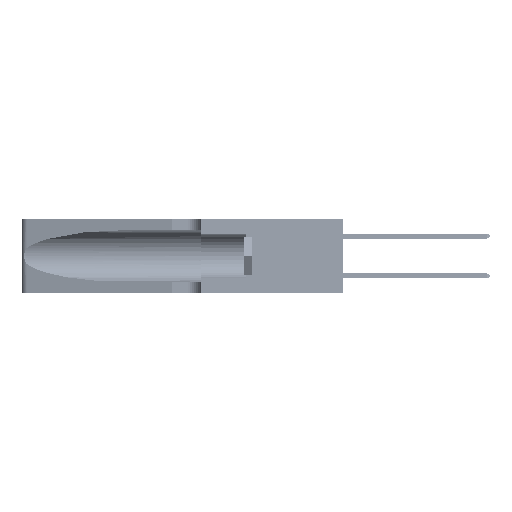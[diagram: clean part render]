
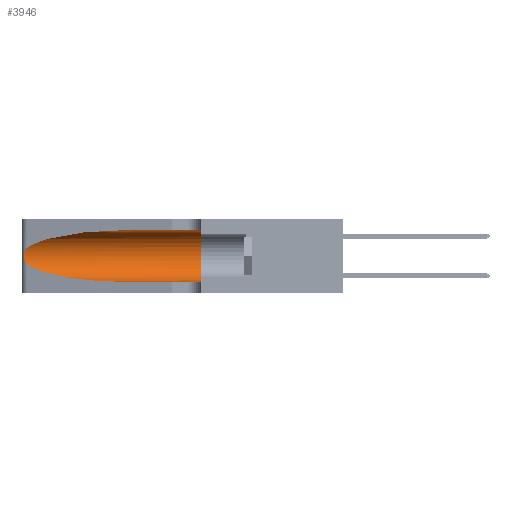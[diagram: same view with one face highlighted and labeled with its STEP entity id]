
A CAD part, left-side view. The second image highlights one B-rep face of the part: STEP entity #3946.
In plain terms, the highlighted cylindrical face has radius 3.308 mm (diameter 6.617 mm), a partial arc.
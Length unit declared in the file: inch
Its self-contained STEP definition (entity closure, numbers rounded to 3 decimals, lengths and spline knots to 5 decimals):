
#882 = DIRECTION ( 'NONE',  ( 0., -1., 0. ) ) ;
#1875 =( BOUNDED_CURVE ( )  B_SPLINE_CURVE ( 3, ( #15972, #15630, #47007, #19424 ),
 .UNSPECIFIED., .F., .F. ) 
 B_SPLINE_CURVE_WITH_KNOTS ( ( 4, 4 ),
 ( 3.44316, 4.71239 ),
 .UNSPECIFIED. ) 
 CURVE ( )  GEOMETRIC_REPRESENTATION_ITEM ( )  RATIONAL_B_SPLINE_CURVE ( ( 1., 0.87, 0.87, 1. ) ) 
 REPRESENTATION_ITEM ( '' )  );
#2103 = CARTESIAN_POINT ( 'NONE',  ( 0.1305, 1.61858, 0.05475 ) ) ;
#2652 = DIRECTION ( 'NONE',  ( 0., -1., 0. ) ) ;
#3429 = CARTESIAN_POINT ( 'NONE',  ( 0.1305, 0.72297, 0.31525 ) ) ;
#3946 = ADVANCED_FACE ( 'NONE', ( #29796 ), #18127, .F. ) ;
#4028 = EDGE_CURVE ( 'NONE', #24841, #21678, #39055, .T. ) ;
#4341 = CARTESIAN_POINT ( 'NONE',  ( 0.25487, 1.22718, 0.22369 ) ) ;
#4496 = VERTEX_POINT ( 'NONE', #13826 ) ;
#5015 = CARTESIAN_POINT ( 'NONE',  ( 0.25789, 1.23486, 0.15765 ) ) ;
#5177 = CARTESIAN_POINT ( 'NONE',  ( 0.1305, 1.61858, 0.31525 ) ) ;
#7983 = EDGE_CURVE ( 'NONE', #21678, #39551, #42183, .T. ) ;
#8445 = CARTESIAN_POINT ( 'NONE',  ( 0.26075, 1.23896, 0.178 ) ) ;
#8957 = CARTESIAN_POINT ( 'NONE',  ( 0.25854, 1.2359, 0.20912 ) ) ;
#11579 = CARTESIAN_POINT ( 'NONE',  ( 0.25487, 1.22718, 0.14631 ) ) ;
#12731 = EDGE_CURVE ( 'NONE', #25545, #4496, #20174, .T. ) ;
#12891 = CARTESIAN_POINT ( 'NONE',  ( 0.25487, 1.22718, 0.22369 ) ) ;
#12968 = CARTESIAN_POINT ( 'NONE',  ( 0.25487, 1.22718, 0.14631 ) ) ;
#13826 = CARTESIAN_POINT ( 'NONE',  ( 0.1305, 0.35, 0.05475 ) ) ;
#13885 = CARTESIAN_POINT ( 'NONE',  ( 0.18966, 0.96281, 0.31525 ) ) ;
#14403 = CARTESIAN_POINT ( 'NONE',  ( 0.1305, 1.61858, 0.185 ) ) ;
#15630 = CARTESIAN_POINT ( 'NONE',  ( 0.2373, 1.15595, 0.08982 ) ) ;
#15972 = CARTESIAN_POINT ( 'NONE',  ( 0.25487, 1.22718, 0.14631 ) ) ;
#16507 = EDGE_CURVE ( 'NONE', #39197, #4496, #48675, .T. ) ;
#17874 = EDGE_LOOP ( 'NONE', ( #23801, #25689, #27011, #43178, #23553, #43185 ) ) ;
#18127 = CYLINDRICAL_SURFACE ( 'NONE', #41851, 0.13025 ) ;
#19424 = CARTESIAN_POINT ( 'NONE',  ( 0.1305, 0.72297, 0.05475 ) ) ;
#19555 = CARTESIAN_POINT ( 'NONE',  ( 0.1305, 0.35, 0.31525 ) ) ;
#20174 = CIRCLE ( 'NONE', #43511, 0.13025 ) ;
#20205 = CARTESIAN_POINT ( 'NONE',  ( 0.26018, 1.23835, 0.19895 ) ) ;
#21096 = DIRECTION ( 'NONE',  ( 0., -1., 0. ) ) ;
#21678 = VERTEX_POINT ( 'NONE', #12891 ) ;
#21803 = CARTESIAN_POINT ( 'NONE',  ( 0.2373, 1.15595, 0.28018 ) ) ;
#23553 = ORIENTED_EDGE ( 'NONE', *, *, #12731, .F. ) ;
#23801 = ORIENTED_EDGE ( 'NONE', *, *, #4028, .T. ) ;
#24009 = CARTESIAN_POINT ( 'NONE',  ( 0.1305, 0.35, 0.185 ) ) ;
#24841 = VERTEX_POINT ( 'NONE', #3429 ) ;
#25545 = VERTEX_POINT ( 'NONE', #19555 ) ;
#25689 = ORIENTED_EDGE ( 'NONE', *, *, #7983, .T. ) ;
#26602 = CARTESIAN_POINT ( 'NONE',  ( 0.25487, 1.22718, 0.22369 ) ) ;
#27011 = ORIENTED_EDGE ( 'NONE', *, *, #45535, .T. ) ;
#28245 = CARTESIAN_POINT ( 'NONE',  ( 0.25555, 1.22994, 0.2215 ) ) ;
#29796 = FACE_OUTER_BOUND ( 'NONE', #17874, .T. ) ;
#30197 = DIRECTION ( 'NONE',  ( 0., 0., -1. ) ) ;
#31852 = CARTESIAN_POINT ( 'NONE',  ( 0.25856, 1.23593, 0.16098 ) ) ;
#32045 = DIRECTION ( 'NONE',  ( 0., 1., 0. ) ) ;
#32225 = DIRECTION ( 'NONE',  ( 0., 0., 1. ) ) ;
#33270 = CARTESIAN_POINT ( 'NONE',  ( 0.1305, 0.72297, 0.05475 ) ) ;
#35949 = CARTESIAN_POINT ( 'NONE',  ( 0.25787, 1.23484, 0.2124 ) ) ;
#36458 = CARTESIAN_POINT ( 'NONE',  ( 0.25639, 1.23186, 0.15144 ) ) ;
#37858 = VECTOR ( 'NONE', #882, 39.37008 ) ;
#39055 =( BOUNDED_CURVE ( )  B_SPLINE_CURVE ( 3, ( #45762, #13885, #21803, #26602 ),
 .UNSPECIFIED., .F., .F. ) 
 B_SPLINE_CURVE_WITH_KNOTS ( ( 4, 4 ),
 ( 1.5708, 2.84003 ),
 .UNSPECIFIED. ) 
 CURVE ( )  GEOMETRIC_REPRESENTATION_ITEM ( )  RATIONAL_B_SPLINE_CURVE ( ( 1., 0.87, 0.87, 1. ) ) 
 REPRESENTATION_ITEM ( '' )  );
#39197 = VERTEX_POINT ( 'NONE', #33270 ) ;
#39551 = VERTEX_POINT ( 'NONE', #11579 ) ;
#39806 = EDGE_CURVE ( 'NONE', #24841, #25545, #48896, .T. ) ;
#40078 = CARTESIAN_POINT ( 'NONE',  ( 0.25555, 1.22993, 0.14849 ) ) ;
#40240 = CARTESIAN_POINT ( 'NONE',  ( 0.26075, 1.23896, 0.19203 ) ) ;
#41851 = AXIS2_PLACEMENT_3D ( 'NONE', #14403, #2652, #30197 ) ;
#41894 = VECTOR ( 'NONE', #21096, 39.37008 ) ;
#42183 = B_SPLINE_CURVE_WITH_KNOTS ( 'NONE', 3,
 ( #4341, #28245, #43664, #35949, #8957, #20205, #40240, #8445, #48124, #31852, #5015, #36458, #40078, #12968 ),
 .UNSPECIFIED., .F., .F.,
 ( 4, 2, 2, 2, 2, 2, 4 ),
 ( 0., 0.00027, 0.00053, 0.00107, 0.0016, 0.00187, 0.00214 ),
 .UNSPECIFIED. ) ;
#43178 = ORIENTED_EDGE ( 'NONE', *, *, #16507, .T. ) ;
#43185 = ORIENTED_EDGE ( 'NONE', *, *, #39806, .F. ) ;
#43511 = AXIS2_PLACEMENT_3D ( 'NONE', #24009, #32045, #32225 ) ;
#43664 = CARTESIAN_POINT ( 'NONE',  ( 0.25639, 1.23184, 0.21858 ) ) ;
#45535 = EDGE_CURVE ( 'NONE', #39551, #39197, #1875, .T. ) ;
#45762 = CARTESIAN_POINT ( 'NONE',  ( 0.1305, 0.72297, 0.31525 ) ) ;
#47007 = CARTESIAN_POINT ( 'NONE',  ( 0.18966, 0.96281, 0.05475 ) ) ;
#48124 = CARTESIAN_POINT ( 'NONE',  ( 0.26017, 1.23833, 0.17102 ) ) ;
#48675 = LINE ( 'NONE', #2103, #41894 ) ;
#48896 = LINE ( 'NONE', #5177, #37858 ) ;
